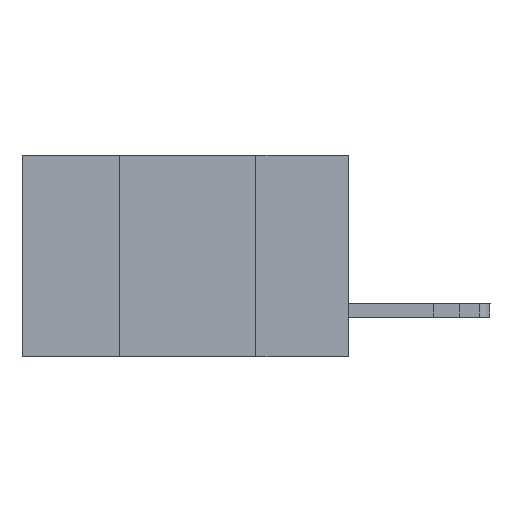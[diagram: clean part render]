
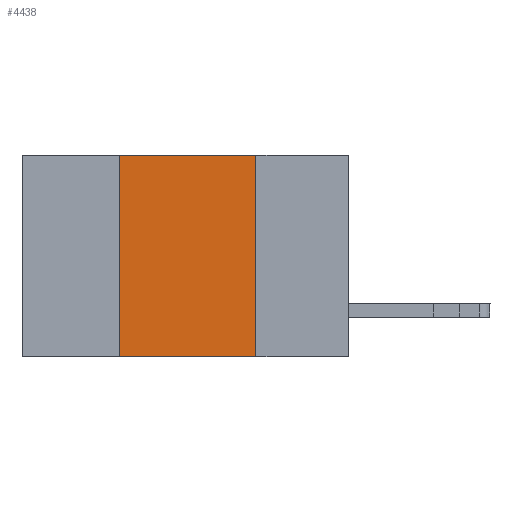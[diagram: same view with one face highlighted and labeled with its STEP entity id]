
A CAD part, left-side view. The second image highlights one B-rep face of the part: STEP entity #4438.
In plain terms, the highlighted planar face has unit normal (-1, 0, 0).
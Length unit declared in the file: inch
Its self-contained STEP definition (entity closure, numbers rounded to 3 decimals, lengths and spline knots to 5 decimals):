
#1254 = VECTOR ( 'NONE', #1920, 39.37008 ) ;
#1696 = LINE ( 'NONE', #2424, #4912 ) ;
#1905 = LINE ( 'NONE', #10932, #12469 ) ;
#1920 = DIRECTION ( 'NONE',  ( 0., 0., 1. ) ) ;
#2026 = DIRECTION ( 'NONE',  ( 0., -1., 0. ) ) ;
#2106 = VECTOR ( 'NONE', #9920, 39.37008 ) ;
#2424 = CARTESIAN_POINT ( 'NONE',  ( 0., 0.6, -0.37 ) ) ;
#2803 = CARTESIAN_POINT ( 'NONE',  ( 0., 0.17, -0.37 ) ) ;
#3563 = AXIS2_PLACEMENT_3D ( 'NONE', #5181, #4168, #7187 ) ;
#3848 = LINE ( 'NONE', #9076, #1254 ) ;
#4168 = DIRECTION ( 'NONE',  ( 1., 0., 0. ) ) ;
#4175 = EDGE_LOOP ( 'NONE', ( #6961, #12414, #5188, #5690 ) ) ;
#4438 = ADVANCED_FACE ( 'NONE', ( #12161 ), #10148, .F. ) ;
#4912 = VECTOR ( 'NONE', #8647, 39.37008 ) ;
#5181 = CARTESIAN_POINT ( 'NONE',  ( 0., 0.6, 0. ) ) ;
#5188 = ORIENTED_EDGE ( 'NONE', *, *, #5228, .F. ) ;
#5228 = EDGE_CURVE ( 'NONE', #9139, #9816, #3848, .T. ) ;
#5690 = ORIENTED_EDGE ( 'NONE', *, *, #7149, .T. ) ;
#5889 = LINE ( 'NONE', #2803, #2106 ) ;
#5980 = CARTESIAN_POINT ( 'NONE',  ( 0., 0.17, 0. ) ) ;
#6073 = EDGE_CURVE ( 'NONE', #10361, #10776, #5889, .T. ) ;
#6570 = CARTESIAN_POINT ( 'NONE',  ( 0., 0.17, -0.37 ) ) ;
#6961 = ORIENTED_EDGE ( 'NONE', *, *, #6073, .F. ) ;
#7149 = EDGE_CURVE ( 'NONE', #9139, #10776, #1696, .T. ) ;
#7187 = DIRECTION ( 'NONE',  ( 0., 0., -1. ) ) ;
#8647 = DIRECTION ( 'NONE',  ( 0., -1., 0. ) ) ;
#8995 = CARTESIAN_POINT ( 'NONE',  ( 0., 0.42, -0.37 ) ) ;
#9076 = CARTESIAN_POINT ( 'NONE',  ( 0., 0.42, -0.37 ) ) ;
#9139 = VERTEX_POINT ( 'NONE', #8995 ) ;
#9816 = VERTEX_POINT ( 'NONE', #10440 ) ;
#9920 = DIRECTION ( 'NONE',  ( 0., 0., -1. ) ) ;
#10148 = PLANE ( 'NONE',  #3563 ) ;
#10361 = VERTEX_POINT ( 'NONE', #5980 ) ;
#10440 = CARTESIAN_POINT ( 'NONE',  ( 0., 0.42, 0. ) ) ;
#10458 = EDGE_CURVE ( 'NONE', #9816, #10361, #1905, .T. ) ;
#10776 = VERTEX_POINT ( 'NONE', #6570 ) ;
#10932 = CARTESIAN_POINT ( 'NONE',  ( 0., 0.6, 0. ) ) ;
#12161 = FACE_OUTER_BOUND ( 'NONE', #4175, .T. ) ;
#12414 = ORIENTED_EDGE ( 'NONE', *, *, #10458, .F. ) ;
#12469 = VECTOR ( 'NONE', #2026, 39.37008 ) ;
